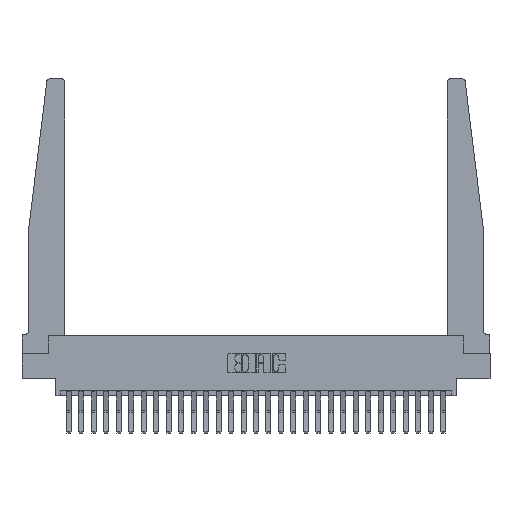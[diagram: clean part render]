
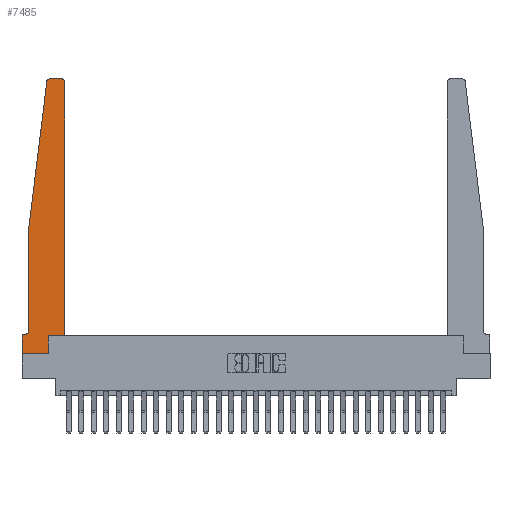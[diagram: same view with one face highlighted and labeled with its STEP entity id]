
A CAD part, top view. The second image highlights one B-rep face of the part: STEP entity #7485.
In plain terms, the highlighted planar face has unit normal (0, 0, 1).
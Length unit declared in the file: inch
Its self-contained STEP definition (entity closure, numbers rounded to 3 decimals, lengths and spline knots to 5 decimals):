
#39 = CARTESIAN_POINT ( 'NONE',  ( 0.425, 2.72, 0.37 ) ) ;
#302 = EDGE_CURVE ( 'NONE', #13369, #17324, #24364, .T. ) ;
#461 = EDGE_CURVE ( 'NONE', #23101, #5122, #18974, .T. ) ;
#591 = VECTOR ( 'NONE', #25704, 39.37008 ) ;
#1188 = DIRECTION ( 'NONE',  ( 1., 0., 0. ) ) ;
#1254 = CARTESIAN_POINT ( 'NONE',  ( 0.2605, 0.18, 0.37 ) ) ;
#1402 = DIRECTION ( 'NONE',  ( 1., 0., 0. ) ) ;
#2019 = DIRECTION ( 'NONE',  ( 1., 0., 0. ) ) ;
#2403 = AXIS2_PLACEMENT_3D ( 'NONE', #17204, #25597, #19813 ) ;
#2493 = EDGE_CURVE ( 'NONE', #4875, #24773, #11101, .T. ) ;
#3498 = CARTESIAN_POINT ( 'NONE',  ( 0.065, 1.25, 0.37 ) ) ;
#3532 = ORIENTED_EDGE ( 'NONE', *, *, #17559, .T. ) ;
#4372 = DIRECTION ( 'NONE',  ( -1., 0., 0. ) ) ;
#4391 = VERTEX_POINT ( 'NONE', #3498 ) ;
#4504 = CARTESIAN_POINT ( 'NONE',  ( 0.25, 2.75, 0.37 ) ) ;
#4875 = VERTEX_POINT ( 'NONE', #24295 ) ;
#4982 = DIRECTION ( 'NONE',  ( 0., -1., 0. ) ) ;
#5122 = VERTEX_POINT ( 'NONE', #23041 ) ;
#5237 = DIRECTION ( 'NONE',  ( 0., 1., 0. ) ) ;
#5486 = VERTEX_POINT ( 'NONE', #23382 ) ;
#5649 = LINE ( 'NONE', #1254, #11585 ) ;
#5929 = VECTOR ( 'NONE', #16915, 39.37008 ) ;
#6070 = LINE ( 'NONE', #11706, #20703 ) ;
#6333 = DIRECTION ( 'NONE',  ( 1., 0., 0. ) ) ;
#6569 = ORIENTED_EDGE ( 'NONE', *, *, #26863, .T. ) ;
#6968 = VERTEX_POINT ( 'NONE', #7592 ) ;
#7310 = LINE ( 'NONE', #23699, #12315 ) ;
#7485 = ADVANCED_FACE ( 'NONE', ( #14938 ), #14527, .T. ) ;
#7592 = CARTESIAN_POINT ( 'NONE',  ( 0.2605, 0., 0.37 ) ) ;
#7967 = ORIENTED_EDGE ( 'NONE', *, *, #13422, .T. ) ;
#8096 = CARTESIAN_POINT ( 'NONE',  ( 0.065, 0.2375, 0.37 ) ) ;
#8672 = DIRECTION ( 'NONE',  ( 0., 0., 1. ) ) ;
#9452 = ORIENTED_EDGE ( 'NONE', *, *, #12422, .T. ) ;
#9515 = LINE ( 'NONE', #14059, #13618 ) ;
#9828 = CARTESIAN_POINT ( 'NONE',  ( 0.24675, 2.72367, 0.37 ) ) ;
#9870 = AXIS2_PLACEMENT_3D ( 'NONE', #20166, #20027, #1188 ) ;
#10060 = CARTESIAN_POINT ( 'NONE',  ( 0.2605, 0.18, 0.37 ) ) ;
#10179 = VECTOR ( 'NONE', #24739, 39.37008 ) ;
#10333 = ORIENTED_EDGE ( 'NONE', *, *, #2493, .T. ) ;
#10725 = EDGE_CURVE ( 'NONE', #4391, #13369, #7310, .T. ) ;
#10850 = ORIENTED_EDGE ( 'NONE', *, *, #10725, .T. ) ;
#11101 = LINE ( 'NONE', #4504, #21485 ) ;
#11283 = AXIS2_PLACEMENT_3D ( 'NONE', #20855, #25111, #2019 ) ;
#11585 = VECTOR ( 'NONE', #5237, 39.37008 ) ;
#11706 = CARTESIAN_POINT ( 'NONE',  ( 0.425, 0.18, 0.37 ) ) ;
#12305 = EDGE_CURVE ( 'NONE', #25896, #5486, #6070, .T. ) ;
#12315 = VECTOR ( 'NONE', #4982, 39.37008 ) ;
#12422 = EDGE_CURVE ( 'NONE', #24773, #23717, #13690, .T. ) ;
#12819 = ORIENTED_EDGE ( 'NONE', *, *, #15844, .T. ) ;
#13093 = CARTESIAN_POINT ( 'NONE',  ( 0., 0.1875, 0.37 ) ) ;
#13369 = VERTEX_POINT ( 'NONE', #8096 ) ;
#13422 = EDGE_CURVE ( 'NONE', #17324, #23101, #22819, .T. ) ;
#13618 = VECTOR ( 'NONE', #20262, 39.37008 ) ;
#13690 = CIRCLE ( 'NONE', #21165, 0.03 ) ;
#14059 = CARTESIAN_POINT ( 'NONE',  ( 0., 0., 0.37 ) ) ;
#14393 = VERTEX_POINT ( 'NONE', #39 ) ;
#14527 = PLANE ( 'NONE',  #11283 ) ;
#14938 = FACE_OUTER_BOUND ( 'NONE', #26999, .T. ) ;
#15844 = EDGE_CURVE ( 'NONE', #5486, #14393, #17048, .T. ) ;
#16489 = ORIENTED_EDGE ( 'NONE', *, *, #461, .T. ) ;
#16915 = DIRECTION ( 'NONE',  ( 0., -1., 0. ) ) ;
#17048 = LINE ( 'NONE', #25438, #591 ) ;
#17204 = CARTESIAN_POINT ( 'NONE',  ( 0.015, 0.2375, 0.37 ) ) ;
#17324 = VERTEX_POINT ( 'NONE', #20952 ) ;
#17559 = EDGE_CURVE ( 'NONE', #5122, #6968, #9515, .T. ) ;
#18000 = EDGE_CURVE ( 'NONE', #6968, #25896, #5649, .T. ) ;
#18974 = LINE ( 'NONE', #26822, #5929 ) ;
#19813 = DIRECTION ( 'NONE',  ( -1., 0., 0. ) ) ;
#20027 = DIRECTION ( 'NONE',  ( 0., 0., 1. ) ) ;
#20040 = CIRCLE ( 'NONE', #9870, 0.03 ) ;
#20166 = CARTESIAN_POINT ( 'NONE',  ( 0.395, 2.72, 0.37 ) ) ;
#20207 = CARTESIAN_POINT ( 'NONE',  ( 0.065, 1.25, 0.37 ) ) ;
#20262 = DIRECTION ( 'NONE',  ( 1., 0., 0. ) ) ;
#20703 = VECTOR ( 'NONE', #1402, 39.37008 ) ;
#20855 = CARTESIAN_POINT ( 'NONE',  ( 0., 0.1875, 0.37 ) ) ;
#20952 = CARTESIAN_POINT ( 'NONE',  ( 0.015, 0.1875, 0.37 ) ) ;
#21165 = AXIS2_PLACEMENT_3D ( 'NONE', #25319, #8672, #6333 ) ;
#21485 = VECTOR ( 'NONE', #4372, 39.37008 ) ;
#21532 = ORIENTED_EDGE ( 'NONE', *, *, #25226, .T. ) ;
#21655 = ORIENTED_EDGE ( 'NONE', *, *, #18000, .T. ) ;
#22533 = ORIENTED_EDGE ( 'NONE', *, *, #12305, .T. ) ;
#22819 = LINE ( 'NONE', #26931, #10179 ) ;
#23041 = CARTESIAN_POINT ( 'NONE',  ( 0., 0., 0.37 ) ) ;
#23101 = VERTEX_POINT ( 'NONE', #13093 ) ;
#23382 = CARTESIAN_POINT ( 'NONE',  ( 0.425, 0.18, 0.37 ) ) ;
#23699 = CARTESIAN_POINT ( 'NONE',  ( 0.065, 1.25, 0.37 ) ) ;
#23717 = VERTEX_POINT ( 'NONE', #9828 ) ;
#24295 = CARTESIAN_POINT ( 'NONE',  ( 0.395, 2.75, 0.37 ) ) ;
#24318 = DIRECTION ( 'NONE',  ( -0.122, -0.992, 0. ) ) ;
#24364 = CIRCLE ( 'NONE', #2403, 0.05 ) ;
#24446 = VECTOR ( 'NONE', #24318, 39.37008 ) ;
#24715 = ORIENTED_EDGE ( 'NONE', *, *, #302, .T. ) ;
#24739 = DIRECTION ( 'NONE',  ( -1., 0., 0. ) ) ;
#24773 = VERTEX_POINT ( 'NONE', #24896 ) ;
#24896 = CARTESIAN_POINT ( 'NONE',  ( 0.27653, 2.75, 0.37 ) ) ;
#25111 = DIRECTION ( 'NONE',  ( 0., 0., 1. ) ) ;
#25226 = EDGE_CURVE ( 'NONE', #14393, #4875, #20040, .T. ) ;
#25319 = CARTESIAN_POINT ( 'NONE',  ( 0.27653, 2.72, 0.37 ) ) ;
#25438 = CARTESIAN_POINT ( 'NONE',  ( 0.425, 0.18, 0.37 ) ) ;
#25597 = DIRECTION ( 'NONE',  ( 0., 0., -1. ) ) ;
#25704 = DIRECTION ( 'NONE',  ( 0., 1., 0. ) ) ;
#25896 = VERTEX_POINT ( 'NONE', #10060 ) ;
#26384 = LINE ( 'NONE', #20207, #24446 ) ;
#26822 = CARTESIAN_POINT ( 'NONE',  ( 0., 0., 0.37 ) ) ;
#26863 = EDGE_CURVE ( 'NONE', #23717, #4391, #26384, .T. ) ;
#26931 = CARTESIAN_POINT ( 'NONE',  ( 0.065, 0.1875, 0.37 ) ) ;
#26999 = EDGE_LOOP ( 'NONE', ( #10333, #9452, #6569, #10850, #24715, #7967, #16489, #3532, #21655, #22533, #12819, #21532 ) ) ;
